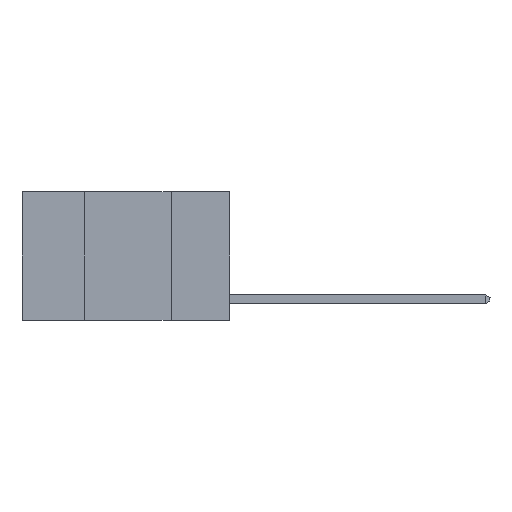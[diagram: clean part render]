
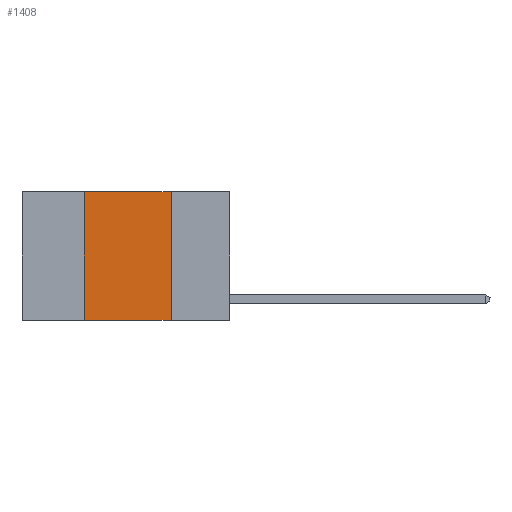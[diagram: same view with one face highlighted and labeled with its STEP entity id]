
A CAD part, left-side view. The second image highlights one B-rep face of the part: STEP entity #1408.
In plain terms, the highlighted planar face has unit normal (-1, 0, 0).
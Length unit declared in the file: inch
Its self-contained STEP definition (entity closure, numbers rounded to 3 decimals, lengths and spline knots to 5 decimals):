
#317 = CARTESIAN_POINT ( 'NONE',  ( 0., 0.6, 0. ) ) ;
#464 = VERTEX_POINT ( 'NONE', #8883 ) ;
#622 = DIRECTION ( 'NONE',  ( 0., -1., 0. ) ) ;
#760 = EDGE_CURVE ( 'NONE', #5109, #3448, #7898, .T. ) ;
#916 = EDGE_CURVE ( 'NONE', #6151, #464, #11990, .T. ) ;
#1408 = ADVANCED_FACE ( 'NONE', ( #12106 ), #9996, .F. ) ;
#2290 = CARTESIAN_POINT ( 'NONE',  ( 0., 0.42, 0. ) ) ;
#2468 = CARTESIAN_POINT ( 'NONE',  ( 0., 0.42, -0.37 ) ) ;
#2511 = DIRECTION ( 'NONE',  ( 1., 0., 0. ) ) ;
#2593 = CARTESIAN_POINT ( 'NONE',  ( 0., 0.6, -0.37 ) ) ;
#3317 = CARTESIAN_POINT ( 'NONE',  ( 0., 0.6, 0. ) ) ;
#3448 = VERTEX_POINT ( 'NONE', #4262 ) ;
#3919 = VECTOR ( 'NONE', #9023, 39.37008 ) ;
#3993 = ORIENTED_EDGE ( 'NONE', *, *, #760, .F. ) ;
#4262 = CARTESIAN_POINT ( 'NONE',  ( 0., 0.17, -0.37 ) ) ;
#4986 = ORIENTED_EDGE ( 'NONE', *, *, #916, .F. ) ;
#5109 = VERTEX_POINT ( 'NONE', #8643 ) ;
#5135 = AXIS2_PLACEMENT_3D ( 'NONE', #317, #2511, #9696 ) ;
#6151 = VERTEX_POINT ( 'NONE', #2468 ) ;
#6426 = LINE ( 'NONE', #3317, #3919 ) ;
#6460 = EDGE_CURVE ( 'NONE', #6151, #3448, #11149, .T. ) ;
#6709 = EDGE_LOOP ( 'NONE', ( #3993, #8137, #4986, #7110 ) ) ;
#6989 = VECTOR ( 'NONE', #9290, 39.37008 ) ;
#7009 = EDGE_CURVE ( 'NONE', #464, #5109, #6426, .T. ) ;
#7110 = ORIENTED_EDGE ( 'NONE', *, *, #6460, .T. ) ;
#7710 = DIRECTION ( 'NONE',  ( 0., 0., 1. ) ) ;
#7898 = LINE ( 'NONE', #9435, #6989 ) ;
#8099 = VECTOR ( 'NONE', #622, 39.37008 ) ;
#8137 = ORIENTED_EDGE ( 'NONE', *, *, #7009, .F. ) ;
#8643 = CARTESIAN_POINT ( 'NONE',  ( 0., 0.17, 0. ) ) ;
#8883 = CARTESIAN_POINT ( 'NONE',  ( 0., 0.42, 0. ) ) ;
#9023 = DIRECTION ( 'NONE',  ( 0., -1., 0. ) ) ;
#9290 = DIRECTION ( 'NONE',  ( 0., 0., -1. ) ) ;
#9435 = CARTESIAN_POINT ( 'NONE',  ( 0., 0.17, 0. ) ) ;
#9633 = VECTOR ( 'NONE', #7710, 39.37008 ) ;
#9696 = DIRECTION ( 'NONE',  ( 0., 0., -1. ) ) ;
#9996 = PLANE ( 'NONE',  #5135 ) ;
#11149 = LINE ( 'NONE', #2593, #8099 ) ;
#11990 = LINE ( 'NONE', #2290, #9633 ) ;
#12106 = FACE_OUTER_BOUND ( 'NONE', #6709, .T. ) ;
